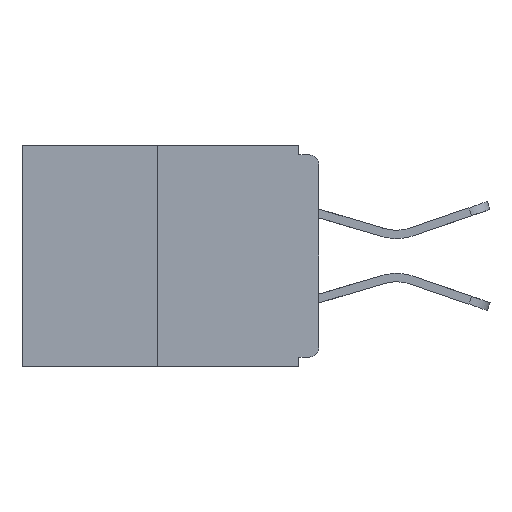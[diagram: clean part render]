
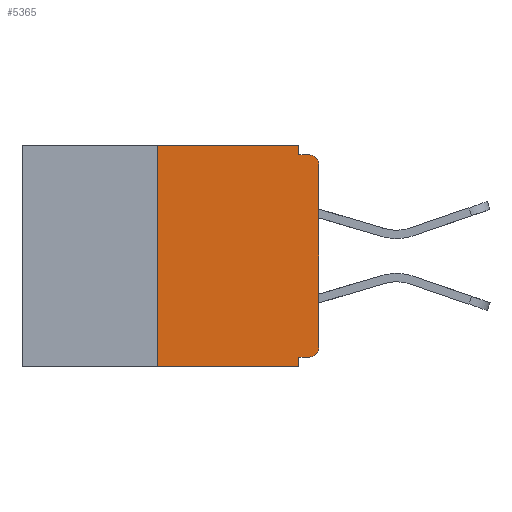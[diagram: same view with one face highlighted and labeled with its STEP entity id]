
A CAD part, left-side view. The second image highlights one B-rep face of the part: STEP entity #5365.
In plain terms, the highlighted planar face has unit normal (-1, 0, 0).
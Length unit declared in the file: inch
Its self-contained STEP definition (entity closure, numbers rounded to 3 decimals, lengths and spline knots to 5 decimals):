
#267 = CIRCLE ( 'NONE', #7517, 0.015 ) ;
#295 = CARTESIAN_POINT ( 'NONE',  ( 0., 0.031, -0.328 ) ) ;
#297 = LINE ( 'NONE', #11928, #10010 ) ;
#477 = ORIENTED_EDGE ( 'NONE', *, *, #16789, .T. ) ;
#886 = CARTESIAN_POINT ( 'NONE',  ( 0., 0., -0.015 ) ) ;
#979 = DIRECTION ( 'NONE',  ( 0., 0., -1. ) ) ;
#1056 = CARTESIAN_POINT ( 'NONE',  ( 0., 0.031, 0. ) ) ;
#1106 = CARTESIAN_POINT ( 'NONE',  ( 0., 0.25, 0. ) ) ;
#1221 = EDGE_CURVE ( 'NONE', #4793, #3820, #297, .T. ) ;
#1238 = ORIENTED_EDGE ( 'NONE', *, *, #10891, .F. ) ;
#1516 = DIRECTION ( 'NONE',  ( -1., 0., 0. ) ) ;
#1683 = DIRECTION ( 'NONE',  ( 0., 0., 1. ) ) ;
#1789 = VECTOR ( 'NONE', #14739, 39.37008 ) ;
#2001 = EDGE_LOOP ( 'NONE', ( #10413, #11871, #5903, #10727, #11138, #17022, #6244, #477, #1238, #16474 ) ) ;
#2378 = VERTEX_POINT ( 'NONE', #5052 ) ;
#2482 = CARTESIAN_POINT ( 'NONE',  ( 0., 0.015, -0.03 ) ) ;
#2817 = CARTESIAN_POINT ( 'NONE',  ( 0., 0.25, -0.343 ) ) ;
#2965 = CARTESIAN_POINT ( 'NONE',  ( 0., 0.015, -0.313 ) ) ;
#3146 = LINE ( 'NONE', #886, #14642 ) ;
#3820 = VERTEX_POINT ( 'NONE', #15525 ) ;
#4186 = AXIS2_PLACEMENT_3D ( 'NONE', #2965, #1516, #15944 ) ;
#4325 = EDGE_CURVE ( 'NONE', #9930, #2378, #12015, .T. ) ;
#4793 = VERTEX_POINT ( 'NONE', #15515 ) ;
#4811 = VERTEX_POINT ( 'NONE', #2817 ) ;
#5052 = CARTESIAN_POINT ( 'NONE',  ( 0., 0.031, -0.343 ) ) ;
#5074 = CIRCLE ( 'NONE', #4186, 0.015 ) ;
#5140 = VECTOR ( 'NONE', #15244, 39.37008 ) ;
#5365 = ADVANCED_FACE ( 'NONE', ( #11525 ), #17208, .F. ) ;
#5442 = CARTESIAN_POINT ( 'NONE',  ( 0., 0.031, 0. ) ) ;
#5903 = ORIENTED_EDGE ( 'NONE', *, *, #9265, .T. ) ;
#5906 = EDGE_CURVE ( 'NONE', #9138, #9930, #18248, .T. ) ;
#6056 = VERTEX_POINT ( 'NONE', #5442 ) ;
#6082 = VERTEX_POINT ( 'NONE', #14015 ) ;
#6121 = LINE ( 'NONE', #6797, #11994 ) ;
#6244 = ORIENTED_EDGE ( 'NONE', *, *, #1221, .T. ) ;
#6680 = EDGE_CURVE ( 'NONE', #6056, #9214, #8080, .T. ) ;
#6797 = CARTESIAN_POINT ( 'NONE',  ( 0., 0.46, 0. ) ) ;
#7173 = LINE ( 'NONE', #12773, #12814 ) ;
#7493 = CARTESIAN_POINT ( 'NONE',  ( 0., 0.031, -0.015 ) ) ;
#7517 = AXIS2_PLACEMENT_3D ( 'NONE', #2482, #13893, #979 ) ;
#7884 = DIRECTION ( 'NONE',  ( 0., -1., 0. ) ) ;
#8052 = CARTESIAN_POINT ( 'NONE',  ( 0., 0.015, -0.328 ) ) ;
#8080 = LINE ( 'NONE', #1056, #5140 ) ;
#9138 = VERTEX_POINT ( 'NONE', #8052 ) ;
#9214 = VERTEX_POINT ( 'NONE', #7493 ) ;
#9265 = EDGE_CURVE ( 'NONE', #4811, #2378, #15199, .T. ) ;
#9419 = VERTEX_POINT ( 'NONE', #1106 ) ;
#9574 = DIRECTION ( 'NONE',  ( 0., -1., 0. ) ) ;
#9930 = VERTEX_POINT ( 'NONE', #295 ) ;
#10010 = VECTOR ( 'NONE', #1683, 39.37008 ) ;
#10240 = CARTESIAN_POINT ( 'NONE',  ( 0., 0.031, -0.343 ) ) ;
#10413 = ORIENTED_EDGE ( 'NONE', *, *, #10576, .F. ) ;
#10443 = VECTOR ( 'NONE', #11559, 39.37008 ) ;
#10493 = CARTESIAN_POINT ( 'NONE',  ( 0., 0.46, 0. ) ) ;
#10576 = EDGE_CURVE ( 'NONE', #9419, #6056, #6121, .T. ) ;
#10727 = ORIENTED_EDGE ( 'NONE', *, *, #4325, .F. ) ;
#10780 = DIRECTION ( 'NONE',  ( 0., -1., 0. ) ) ;
#10891 = EDGE_CURVE ( 'NONE', #9214, #6082, #3146, .T. ) ;
#11138 = ORIENTED_EDGE ( 'NONE', *, *, #5906, .F. ) ;
#11525 = FACE_OUTER_BOUND ( 'NONE', #2001, .T. ) ;
#11559 = DIRECTION ( 'NONE',  ( 0., 0., -1. ) ) ;
#11871 = ORIENTED_EDGE ( 'NONE', *, *, #12042, .F. ) ;
#11928 = CARTESIAN_POINT ( 'NONE',  ( 0., 0., 0. ) ) ;
#11994 = VECTOR ( 'NONE', #9574, 39.37008 ) ;
#12015 = LINE ( 'NONE', #10240, #10443 ) ;
#12042 = EDGE_CURVE ( 'NONE', #4811, #9419, #7173, .T. ) ;
#12503 = VECTOR ( 'NONE', #10780, 39.37008 ) ;
#12773 = CARTESIAN_POINT ( 'NONE',  ( 0., 0.25, 0. ) ) ;
#12814 = VECTOR ( 'NONE', #14151, 39.37008 ) ;
#13003 = AXIS2_PLACEMENT_3D ( 'NONE', #10493, #17459, #14606 ) ;
#13893 = DIRECTION ( 'NONE',  ( -1., 0., 0. ) ) ;
#13942 = EDGE_CURVE ( 'NONE', #9138, #4793, #5074, .T. ) ;
#14015 = CARTESIAN_POINT ( 'NONE',  ( 0., 0.015, -0.015 ) ) ;
#14151 = DIRECTION ( 'NONE',  ( 0., 0., 1. ) ) ;
#14606 = DIRECTION ( 'NONE',  ( 0., 0., -1. ) ) ;
#14642 = VECTOR ( 'NONE', #7884, 39.37008 ) ;
#14739 = DIRECTION ( 'NONE',  ( 0., 1., 0. ) ) ;
#15199 = LINE ( 'NONE', #18122, #12503 ) ;
#15244 = DIRECTION ( 'NONE',  ( 0., 0., -1. ) ) ;
#15515 = CARTESIAN_POINT ( 'NONE',  ( 0., 0., -0.313 ) ) ;
#15525 = CARTESIAN_POINT ( 'NONE',  ( 0., 0., -0.03 ) ) ;
#15944 = DIRECTION ( 'NONE',  ( 0., 0., -1. ) ) ;
#16474 = ORIENTED_EDGE ( 'NONE', *, *, #6680, .F. ) ;
#16789 = EDGE_CURVE ( 'NONE', #3820, #6082, #267, .T. ) ;
#17022 = ORIENTED_EDGE ( 'NONE', *, *, #13942, .T. ) ;
#17208 = PLANE ( 'NONE',  #13003 ) ;
#17459 = DIRECTION ( 'NONE',  ( 1., 0., 0. ) ) ;
#17478 = CARTESIAN_POINT ( 'NONE',  ( 0., 0., -0.328 ) ) ;
#18122 = CARTESIAN_POINT ( 'NONE',  ( 0., 0.46, -0.343 ) ) ;
#18248 = LINE ( 'NONE', #17478, #1789 ) ;
